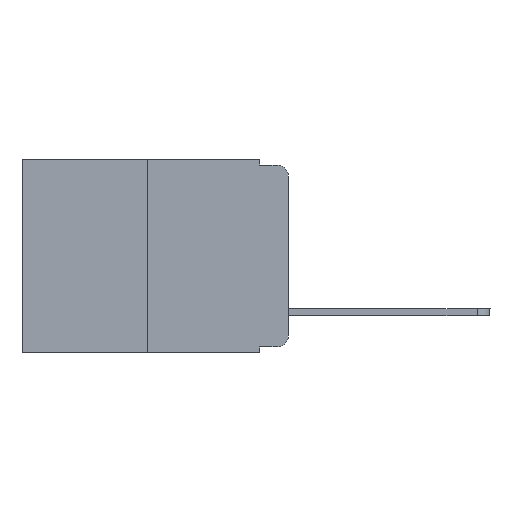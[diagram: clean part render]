
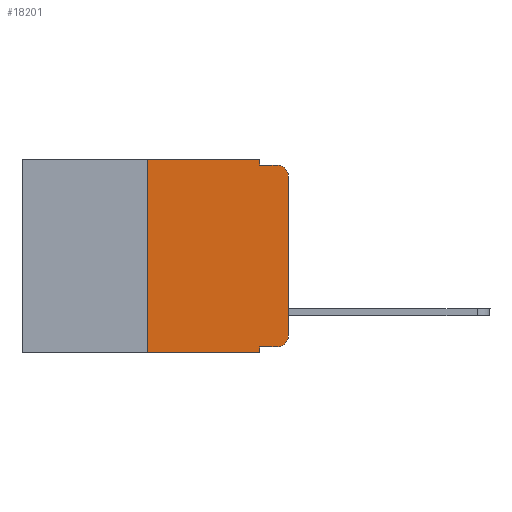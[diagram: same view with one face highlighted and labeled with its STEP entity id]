
A CAD part, left-side view. The second image highlights one B-rep face of the part: STEP entity #18201.
In plain terms, the highlighted planar face has unit normal (-1, 0, 0).
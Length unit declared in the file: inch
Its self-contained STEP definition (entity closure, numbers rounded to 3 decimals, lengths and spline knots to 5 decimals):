
#172 = ORIENTED_EDGE ( 'NONE', *, *, #14249, .F. ) ;
#241 = CARTESIAN_POINT ( 'NONE',  ( 0., 0.02, -0.333 ) ) ;
#355 = CARTESIAN_POINT ( 'NONE',  ( 0., 0.051, 0. ) ) ;
#727 = CARTESIAN_POINT ( 'NONE',  ( 0., 0., 0. ) ) ;
#943 = CARTESIAN_POINT ( 'NONE',  ( 0., 0.473, 0. ) ) ;
#961 = VERTEX_POINT ( 'NONE', #23037 ) ;
#1004 = CARTESIAN_POINT ( 'NONE',  ( 0., 0.473, 0. ) ) ;
#1131 = FACE_OUTER_BOUND ( 'NONE', #2781, .T. ) ;
#1339 = AXIS2_PLACEMENT_3D ( 'NONE', #1004, #10242, #20548 ) ;
#1693 = CARTESIAN_POINT ( 'NONE',  ( 0., 0., -0.03 ) ) ;
#2229 = DIRECTION ( 'NONE',  ( 0., 0., 1. ) ) ;
#2247 = VECTOR ( 'NONE', #3816, 39.37008 ) ;
#2468 = LINE ( 'NONE', #9878, #15594 ) ;
#2637 = VERTEX_POINT ( 'NONE', #10728 ) ;
#2781 = EDGE_LOOP ( 'NONE', ( #21108, #10108, #172, #12568, #11077, #15747, #2842, #15772, #21695, #15216 ) ) ;
#2842 = ORIENTED_EDGE ( 'NONE', *, *, #15763, .T. ) ;
#2918 = EDGE_CURVE ( 'NONE', #7883, #7025, #2468, .T. ) ;
#2986 = VERTEX_POINT ( 'NONE', #21432 ) ;
#3218 = VECTOR ( 'NONE', #16048, 39.37008 ) ;
#3600 = VECTOR ( 'NONE', #22265, 39.37008 ) ;
#3816 = DIRECTION ( 'NONE',  ( 0., 0., -1. ) ) ;
#3875 = DIRECTION ( 'NONE',  ( -1., 0., 0. ) ) ;
#3902 = AXIS2_PLACEMENT_3D ( 'NONE', #7409, #3875, #20077 ) ;
#5170 = CIRCLE ( 'NONE', #18286, 0.02 ) ;
#5990 = CARTESIAN_POINT ( 'NONE',  ( 0., 0.25, 0. ) ) ;
#6009 = CARTESIAN_POINT ( 'NONE',  ( 0., 0.051, -0.01 ) ) ;
#6360 = VERTEX_POINT ( 'NONE', #6846 ) ;
#6752 = CARTESIAN_POINT ( 'NONE',  ( 0., 0.473, -0.343 ) ) ;
#6846 = CARTESIAN_POINT ( 'NONE',  ( 0., 0.051, 0. ) ) ;
#7025 = VERTEX_POINT ( 'NONE', #241 ) ;
#7347 = DIRECTION ( 'NONE',  ( -1., 0., 0. ) ) ;
#7409 = CARTESIAN_POINT ( 'NONE',  ( 0., 0.02, -0.03 ) ) ;
#7540 = VERTEX_POINT ( 'NONE', #15112 ) ;
#7883 = VERTEX_POINT ( 'NONE', #19173 ) ;
#9171 = VECTOR ( 'NONE', #21410, 39.37008 ) ;
#9176 = EDGE_CURVE ( 'NONE', #6360, #2986, #15449, .T. ) ;
#9878 = CARTESIAN_POINT ( 'NONE',  ( 0., 0.051, -0.333 ) ) ;
#10108 = ORIENTED_EDGE ( 'NONE', *, *, #11706, .T. ) ;
#10242 = DIRECTION ( 'NONE',  ( 1., 0., 0. ) ) ;
#10527 = CARTESIAN_POINT ( 'NONE',  ( 0., 0., -0.313 ) ) ;
#10728 = CARTESIAN_POINT ( 'NONE',  ( 0., 0.25, 0. ) ) ;
#11077 = ORIENTED_EDGE ( 'NONE', *, *, #19008, .F. ) ;
#11085 = LINE ( 'NONE', #6752, #3218 ) ;
#11706 = EDGE_CURVE ( 'NONE', #18954, #7540, #18967, .T. ) ;
#11941 = VERTEX_POINT ( 'NONE', #14981 ) ;
#12568 = ORIENTED_EDGE ( 'NONE', *, *, #9176, .F. ) ;
#12711 = EDGE_CURVE ( 'NONE', #961, #2637, #14804, .T. ) ;
#13604 = VECTOR ( 'NONE', #18947, 39.37008 ) ;
#13939 = VECTOR ( 'NONE', #2229, 39.37008 ) ;
#14249 = EDGE_CURVE ( 'NONE', #2986, #7540, #22575, .T. ) ;
#14691 = DIRECTION ( 'NONE',  ( 0., 0., -1. ) ) ;
#14804 = LINE ( 'NONE', #5990, #13939 ) ;
#14965 = PLANE ( 'NONE',  #1339 ) ;
#14981 = CARTESIAN_POINT ( 'NONE',  ( 0., 0.051, -0.343 ) ) ;
#15078 = EDGE_CURVE ( 'NONE', #7883, #11941, #18646, .T. ) ;
#15112 = CARTESIAN_POINT ( 'NONE',  ( 0., 0.02, -0.01 ) ) ;
#15216 = ORIENTED_EDGE ( 'NONE', *, *, #15849, .T. ) ;
#15228 = DIRECTION ( 'NONE',  ( 0., -1., 0. ) ) ;
#15449 = LINE ( 'NONE', #21013, #2247 ) ;
#15594 = VECTOR ( 'NONE', #17226, 39.37008 ) ;
#15747 = ORIENTED_EDGE ( 'NONE', *, *, #12711, .F. ) ;
#15763 = EDGE_CURVE ( 'NONE', #961, #11941, #11085, .T. ) ;
#15772 = ORIENTED_EDGE ( 'NONE', *, *, #15078, .F. ) ;
#15849 = EDGE_CURVE ( 'NONE', #7025, #17087, #5170, .T. ) ;
#15941 = CARTESIAN_POINT ( 'NONE',  ( 0., 0.02, -0.313 ) ) ;
#16048 = DIRECTION ( 'NONE',  ( 0., -1., 0. ) ) ;
#17087 = VERTEX_POINT ( 'NONE', #10527 ) ;
#17226 = DIRECTION ( 'NONE',  ( 0., -1., 0. ) ) ;
#18201 = ADVANCED_FACE ( 'NONE', ( #1131 ), #14965, .F. ) ;
#18286 = AXIS2_PLACEMENT_3D ( 'NONE', #15941, #7347, #14691 ) ;
#18646 = LINE ( 'NONE', #355, #3600 ) ;
#18947 = DIRECTION ( 'NONE',  ( 0., -1., 0. ) ) ;
#18954 = VERTEX_POINT ( 'NONE', #1693 ) ;
#18967 = CIRCLE ( 'NONE', #3902, 0.02 ) ;
#19008 = EDGE_CURVE ( 'NONE', #2637, #6360, #22624, .T. ) ;
#19173 = CARTESIAN_POINT ( 'NONE',  ( 0., 0.051, -0.333 ) ) ;
#20077 = DIRECTION ( 'NONE',  ( 0., 0., -1. ) ) ;
#20548 = DIRECTION ( 'NONE',  ( 0., 0., -1. ) ) ;
#21013 = CARTESIAN_POINT ( 'NONE',  ( 0., 0.051, 0. ) ) ;
#21108 = ORIENTED_EDGE ( 'NONE', *, *, #22284, .T. ) ;
#21181 = LINE ( 'NONE', #727, #9171 ) ;
#21410 = DIRECTION ( 'NONE',  ( 0., 0., 1. ) ) ;
#21432 = CARTESIAN_POINT ( 'NONE',  ( 0., 0.051, -0.01 ) ) ;
#21695 = ORIENTED_EDGE ( 'NONE', *, *, #2918, .T. ) ;
#22216 = VECTOR ( 'NONE', #15228, 39.37008 ) ;
#22265 = DIRECTION ( 'NONE',  ( 0., 0., -1. ) ) ;
#22284 = EDGE_CURVE ( 'NONE', #17087, #18954, #21181, .T. ) ;
#22575 = LINE ( 'NONE', #6009, #13604 ) ;
#22624 = LINE ( 'NONE', #943, #22216 ) ;
#23037 = CARTESIAN_POINT ( 'NONE',  ( 0., 0.25, -0.343 ) ) ;
